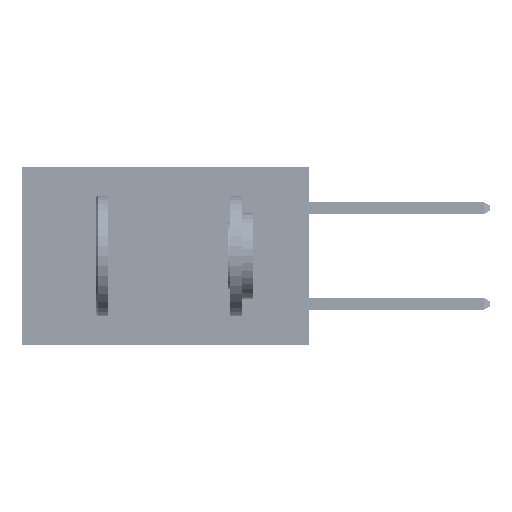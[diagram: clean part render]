
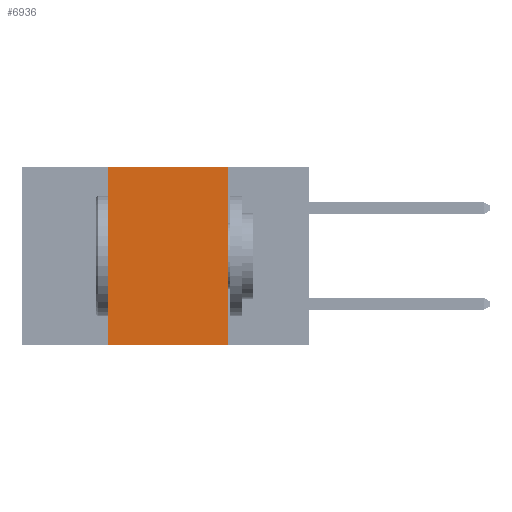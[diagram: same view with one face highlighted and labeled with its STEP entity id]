
A CAD part, left-side view. The second image highlights one B-rep face of the part: STEP entity #6936.
In plain terms, the highlighted planar face has unit normal (-1, 0, 0).
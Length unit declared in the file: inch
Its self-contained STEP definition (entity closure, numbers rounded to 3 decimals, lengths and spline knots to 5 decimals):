
#757 = CARTESIAN_POINT ( 'NONE',  ( 0., 0.42, -0.37 ) ) ;
#2264 = EDGE_CURVE ( 'NONE', #30363, #15957, #32615, .T. ) ;
#3611 = DIRECTION ( 'NONE',  ( 0., 0., -1. ) ) ;
#4587 = LINE ( 'NONE', #8265, #25077 ) ;
#6936 = ADVANCED_FACE ( 'NONE', ( #18551 ), #7361, .F. ) ;
#7021 = DIRECTION ( 'NONE',  ( 1., 0., 0. ) ) ;
#7361 = PLANE ( 'NONE',  #44152 ) ;
#8265 = CARTESIAN_POINT ( 'NONE',  ( 0., 0.6, 0. ) ) ;
#8871 = DIRECTION ( 'NONE',  ( 0., -1., 0. ) ) ;
#9257 = EDGE_CURVE ( 'NONE', #11705, #30363, #4587, .T. ) ;
#11705 = VERTEX_POINT ( 'NONE', #47016 ) ;
#14026 = CARTESIAN_POINT ( 'NONE',  ( 0., 0.17, -0.37 ) ) ;
#14247 = CARTESIAN_POINT ( 'NONE',  ( 0., 0.17, 0. ) ) ;
#15957 = VERTEX_POINT ( 'NONE', #14026 ) ;
#16279 = VECTOR ( 'NONE', #21123, 39.37008 ) ;
#17178 = VERTEX_POINT ( 'NONE', #757 ) ;
#18551 = FACE_OUTER_BOUND ( 'NONE', #50007, .T. ) ;
#18795 = DIRECTION ( 'NONE',  ( 0., 0., -1. ) ) ;
#19155 = CARTESIAN_POINT ( 'NONE',  ( 0., 0.6, 0. ) ) ;
#19398 = CARTESIAN_POINT ( 'NONE',  ( 0., 0.17, 0. ) ) ;
#21123 = DIRECTION ( 'NONE',  ( 0., 0., 1. ) ) ;
#22254 = EDGE_CURVE ( 'NONE', #17178, #11705, #26834, .T. ) ;
#25077 = VECTOR ( 'NONE', #40279, 39.37008 ) ;
#25702 = ORIENTED_EDGE ( 'NONE', *, *, #2264, .F. ) ;
#26834 = LINE ( 'NONE', #49021, #16279 ) ;
#28458 = CARTESIAN_POINT ( 'NONE',  ( 0., 0.6, -0.37 ) ) ;
#30363 = VERTEX_POINT ( 'NONE', #14247 ) ;
#32314 = ORIENTED_EDGE ( 'NONE', *, *, #9257, .F. ) ;
#32615 = LINE ( 'NONE', #19398, #34491 ) ;
#34491 = VECTOR ( 'NONE', #3611, 39.37008 ) ;
#36002 = ORIENTED_EDGE ( 'NONE', *, *, #46417, .T. ) ;
#39306 = VECTOR ( 'NONE', #8871, 39.37008 ) ;
#40279 = DIRECTION ( 'NONE',  ( 0., -1., 0. ) ) ;
#40989 = ORIENTED_EDGE ( 'NONE', *, *, #22254, .F. ) ;
#44152 = AXIS2_PLACEMENT_3D ( 'NONE', #19155, #7021, #18795 ) ;
#46119 = LINE ( 'NONE', #28458, #39306 ) ;
#46417 = EDGE_CURVE ( 'NONE', #17178, #15957, #46119, .T. ) ;
#47016 = CARTESIAN_POINT ( 'NONE',  ( 0., 0.42, 0. ) ) ;
#49021 = CARTESIAN_POINT ( 'NONE',  ( 0., 0.42, 0. ) ) ;
#50007 = EDGE_LOOP ( 'NONE', ( #25702, #32314, #40989, #36002 ) ) ;
